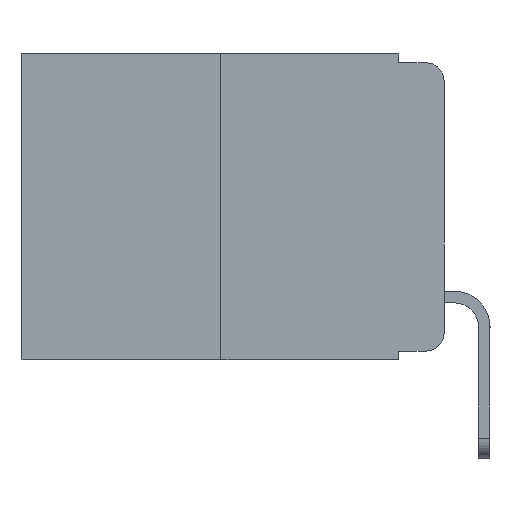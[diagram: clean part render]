
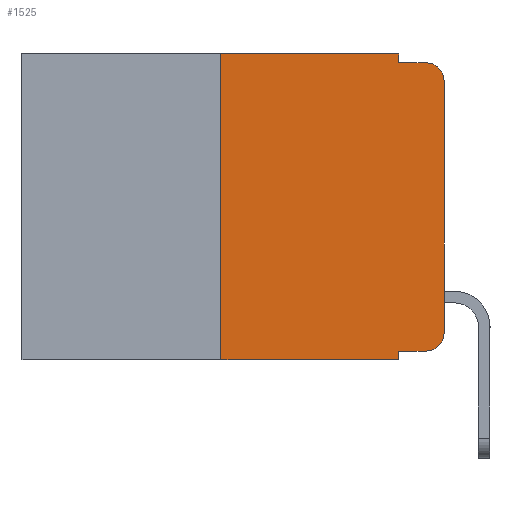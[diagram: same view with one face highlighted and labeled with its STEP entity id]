
A CAD part, left-side view. The second image highlights one B-rep face of the part: STEP entity #1525.
In plain terms, the highlighted planar face has unit normal (-1, 0, 0).
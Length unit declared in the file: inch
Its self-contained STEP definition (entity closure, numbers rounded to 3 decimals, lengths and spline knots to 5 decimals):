
#431 = VERTEX_POINT ( 'NONE', #15093 ) ;
#760 = VERTEX_POINT ( 'NONE', #13141 ) ;
#1011 = DIRECTION ( 'NONE',  ( 0., 0., -1. ) ) ;
#1070 = VECTOR ( 'NONE', #11348, 39.37008 ) ;
#1159 = DIRECTION ( 'NONE',  ( 0., 0., 1. ) ) ;
#1291 = PLANE ( 'NONE',  #7233 ) ;
#1452 = LINE ( 'NONE', #15582, #9177 ) ;
#1525 = ADVANCED_FACE ( 'NONE', ( #10260 ), #1291, .F. ) ;
#2152 = DIRECTION ( 'NONE',  ( -1., 0., 0. ) ) ;
#2753 = VERTEX_POINT ( 'NONE', #5943 ) ;
#2760 = VERTEX_POINT ( 'NONE', #12160 ) ;
#3651 = VERTEX_POINT ( 'NONE', #6378 ) ;
#3871 = CARTESIAN_POINT ( 'NONE',  ( 0., 0.051, 0. ) ) ;
#3957 = AXIS2_PLACEMENT_3D ( 'NONE', #14331, #2152, #1011 ) ;
#4479 = ORIENTED_EDGE ( 'NONE', *, *, #6092, .T. ) ;
#4598 = VERTEX_POINT ( 'NONE', #9951 ) ;
#4718 = VECTOR ( 'NONE', #10444, 39.37008 ) ;
#4723 = ORIENTED_EDGE ( 'NONE', *, *, #6048, .T. ) ;
#4993 = VERTEX_POINT ( 'NONE', #14249 ) ;
#5189 = ORIENTED_EDGE ( 'NONE', *, *, #5831, .F. ) ;
#5373 = LINE ( 'NONE', #10045, #14941 ) ;
#5423 = ORIENTED_EDGE ( 'NONE', *, *, #5994, .F. ) ;
#5461 = CARTESIAN_POINT ( 'NONE',  ( 0., 0.473, 0. ) ) ;
#5515 = ORIENTED_EDGE ( 'NONE', *, *, #11080, .F. ) ;
#5553 = EDGE_CURVE ( 'NONE', #14498, #4598, #10050, .T. ) ;
#5614 = EDGE_CURVE ( 'NONE', #2760, #2753, #12097, .T. ) ;
#5717 = CARTESIAN_POINT ( 'NONE',  ( 0., 0.25, -0.343 ) ) ;
#5740 = EDGE_CURVE ( 'NONE', #2760, #4993, #7615, .T. ) ;
#5831 = EDGE_CURVE ( 'NONE', #431, #11888, #5373, .T. ) ;
#5870 = DIRECTION ( 'NONE',  ( 1., 0., 0. ) ) ;
#5908 = ORIENTED_EDGE ( 'NONE', *, *, #5553, .F. ) ;
#5935 = EDGE_CURVE ( 'NONE', #4993, #3651, #10759, .T. ) ;
#5943 = CARTESIAN_POINT ( 'NONE',  ( 0., 0.051, -0.343 ) ) ;
#5994 = EDGE_CURVE ( 'NONE', #11549, #431, #13133, .T. ) ;
#6004 = CARTESIAN_POINT ( 'NONE',  ( 0., 0.02, -0.03 ) ) ;
#6048 = EDGE_CURVE ( 'NONE', #760, #11888, #8891, .T. ) ;
#6092 = EDGE_CURVE ( 'NONE', #3651, #760, #8451, .T. ) ;
#6246 = ORIENTED_EDGE ( 'NONE', *, *, #7878, .T. ) ;
#6264 = ORIENTED_EDGE ( 'NONE', *, *, #5614, .F. ) ;
#6378 = CARTESIAN_POINT ( 'NONE',  ( 0., 0., -0.313 ) ) ;
#6560 = ORIENTED_EDGE ( 'NONE', *, *, #5740, .T. ) ;
#6905 = ORIENTED_EDGE ( 'NONE', *, *, #5935, .T. ) ;
#7233 = AXIS2_PLACEMENT_3D ( 'NONE', #5461, #5870, #16817 ) ;
#7292 = LINE ( 'NONE', #8994, #16830 ) ;
#7615 = LINE ( 'NONE', #14072, #16737 ) ;
#7878 = EDGE_CURVE ( 'NONE', #14498, #2753, #7292, .T. ) ;
#8451 = LINE ( 'NONE', #9036, #4718 ) ;
#8874 = DIRECTION ( 'NONE',  ( 0., -1., 0. ) ) ;
#8891 = CIRCLE ( 'NONE', #10353, 0.02 ) ;
#8928 = DIRECTION ( 'NONE',  ( -1., 0., 0. ) ) ;
#8994 = CARTESIAN_POINT ( 'NONE',  ( 0., 0.473, -0.343 ) ) ;
#9036 = CARTESIAN_POINT ( 'NONE',  ( 0., 0., 0. ) ) ;
#9091 = CARTESIAN_POINT ( 'NONE',  ( 0., 0.051, 0. ) ) ;
#9177 = VECTOR ( 'NONE', #10929, 39.37008 ) ;
#9267 = DIRECTION ( 'NONE',  ( 0., 0., -1. ) ) ;
#9632 = CARTESIAN_POINT ( 'NONE',  ( 0., 0.051, 0. ) ) ;
#9951 = CARTESIAN_POINT ( 'NONE',  ( 0., 0.25, 0. ) ) ;
#10032 = VECTOR ( 'NONE', #9267, 39.37008 ) ;
#10045 = CARTESIAN_POINT ( 'NONE',  ( 0., 0.051, -0.01 ) ) ;
#10050 = LINE ( 'NONE', #16305, #15842 ) ;
#10260 = FACE_OUTER_BOUND ( 'NONE', #13060, .T. ) ;
#10353 = AXIS2_PLACEMENT_3D ( 'NONE', #6004, #8928, #14469 ) ;
#10444 = DIRECTION ( 'NONE',  ( 0., 0., 1. ) ) ;
#10759 = CIRCLE ( 'NONE', #3957, 0.02 ) ;
#10929 = DIRECTION ( 'NONE',  ( 0., -1., 0. ) ) ;
#11080 = EDGE_CURVE ( 'NONE', #4598, #11549, #1452, .T. ) ;
#11348 = DIRECTION ( 'NONE',  ( 0., 0., -1. ) ) ;
#11549 = VERTEX_POINT ( 'NONE', #3871 ) ;
#11888 = VERTEX_POINT ( 'NONE', #12315 ) ;
#12006 = DIRECTION ( 'NONE',  ( 0., -1., 0. ) ) ;
#12097 = LINE ( 'NONE', #9632, #1070 ) ;
#12160 = CARTESIAN_POINT ( 'NONE',  ( 0., 0.051, -0.333 ) ) ;
#12315 = CARTESIAN_POINT ( 'NONE',  ( 0., 0.02, -0.01 ) ) ;
#13060 = EDGE_LOOP ( 'NONE', ( #4479, #4723, #5189, #5423, #5515, #5908, #6246, #6264, #6560, #6905 ) ) ;
#13066 = DIRECTION ( 'NONE',  ( 0., -1., 0. ) ) ;
#13133 = LINE ( 'NONE', #9091, #10032 ) ;
#13141 = CARTESIAN_POINT ( 'NONE',  ( 0., 0., -0.03 ) ) ;
#14072 = CARTESIAN_POINT ( 'NONE',  ( 0., 0.051, -0.333 ) ) ;
#14249 = CARTESIAN_POINT ( 'NONE',  ( 0., 0.02, -0.333 ) ) ;
#14331 = CARTESIAN_POINT ( 'NONE',  ( 0., 0.02, -0.313 ) ) ;
#14469 = DIRECTION ( 'NONE',  ( 0., 0., -1. ) ) ;
#14498 = VERTEX_POINT ( 'NONE', #5717 ) ;
#14941 = VECTOR ( 'NONE', #13066, 39.37008 ) ;
#15093 = CARTESIAN_POINT ( 'NONE',  ( 0., 0.051, -0.01 ) ) ;
#15582 = CARTESIAN_POINT ( 'NONE',  ( 0., 0.473, 0. ) ) ;
#15842 = VECTOR ( 'NONE', #1159, 39.37008 ) ;
#16305 = CARTESIAN_POINT ( 'NONE',  ( 0., 0.25, 0. ) ) ;
#16737 = VECTOR ( 'NONE', #12006, 39.37008 ) ;
#16817 = DIRECTION ( 'NONE',  ( 0., 0., -1. ) ) ;
#16830 = VECTOR ( 'NONE', #8874, 39.37008 ) ;
